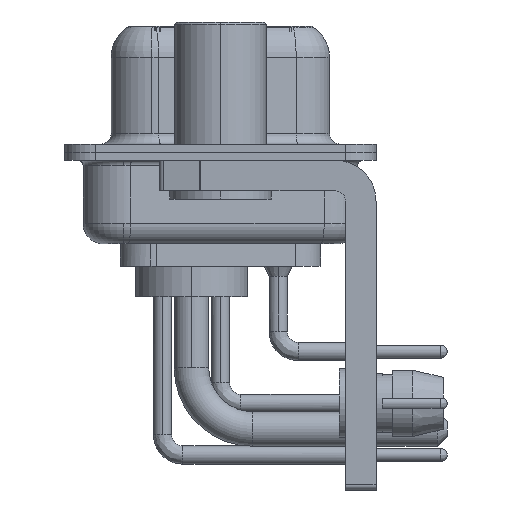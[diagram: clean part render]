
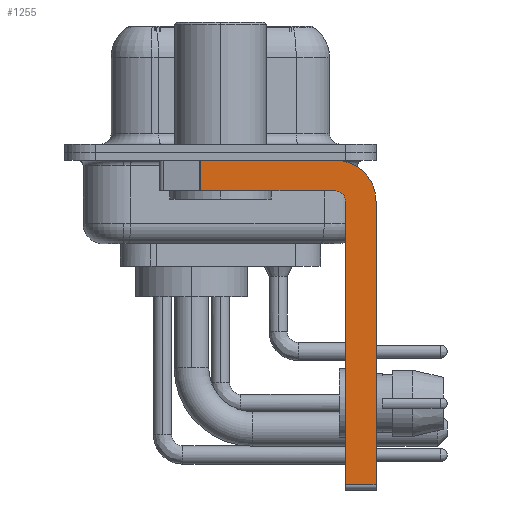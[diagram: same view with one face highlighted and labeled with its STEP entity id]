
A CAD part, left-side view. The second image highlights one B-rep face of the part: STEP entity #1255.
In plain terms, the highlighted planar face has unit normal (-1, 0, 0).
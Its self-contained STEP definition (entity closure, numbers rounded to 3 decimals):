
#630 = ORIENTED_EDGE ( 'NONE', *, *, #1553, .F. ) ;
#1255 = ADVANCED_FACE ( 'NONE', ( #2744 ), #27591, .F. ) ;
#1553 = EDGE_CURVE ( 'NONE', #31914, #4604, #4413, .T. ) ;
#1892 = CARTESIAN_POINT ( 'NONE',  ( -2.9, 0.978, -1.9 ) ) ;
#1980 = EDGE_CURVE ( 'NONE', #17099, #31914, #19887, .T. ) ;
#2428 = CARTESIAN_POINT ( 'NONE',  ( -2.9, 0.978, -0.4 ) ) ;
#2476 = LINE ( 'NONE', #30047, #4962 ) ;
#2685 = AXIS2_PLACEMENT_3D ( 'NONE', #12939, #18265, #9809 ) ;
#2696 = DIRECTION ( 'NONE',  ( 0., 0., -1. ) ) ;
#2702 = VECTOR ( 'NONE', #23407, 1000. ) ;
#2744 = FACE_OUTER_BOUND ( 'NONE', #30537, .T. ) ;
#4413 = CIRCLE ( 'NONE', #2685, 2. ) ;
#4604 = VERTEX_POINT ( 'NONE', #15969 ) ;
#4962 = VECTOR ( 'NONE', #35711, 1000. ) ;
#5064 = LINE ( 'NONE', #13667, #18791 ) ;
#5450 = ORIENTED_EDGE ( 'NONE', *, *, #23052, .F. ) ;
#5468 = EDGE_CURVE ( 'NONE', #18731, #22266, #2476, .T. ) ;
#5472 = DIRECTION ( 'NONE',  ( 0., 0., -1. ) ) ;
#5540 = EDGE_CURVE ( 'NONE', #31088, #14225, #25123, .T. ) ;
#5852 = ORIENTED_EDGE ( 'NONE', *, *, #6042, .F. ) ;
#5921 = DIRECTION ( 'NONE',  ( 0., -1., 0. ) ) ;
#5974 = CARTESIAN_POINT ( 'NONE',  ( -2.9, 3., -0.4 ) ) ;
#6042 = EDGE_CURVE ( 'NONE', #31088, #7208, #34734, .T. ) ;
#6273 = EDGE_CURVE ( 'NONE', #17099, #22266, #23935, .T. ) ;
#7134 = CARTESIAN_POINT ( 'NONE',  ( -2.9, -5.65, -1.9 ) ) ;
#7208 = VERTEX_POINT ( 'NONE', #22126 ) ;
#9035 = CARTESIAN_POINT ( 'NONE',  ( -2.9, -5.65, -16.35 ) ) ;
#9809 = DIRECTION ( 'NONE',  ( 0., 0., -1. ) ) ;
#10960 = CARTESIAN_POINT ( 'NONE',  ( -2.9, -6.15, -16.35 ) ) ;
#11982 = EDGE_CURVE ( 'NONE', #4604, #14225, #5064, .T. ) ;
#12939 = CARTESIAN_POINT ( 'NONE',  ( -2.9, -5.65, -2.4 ) ) ;
#13667 = CARTESIAN_POINT ( 'NONE',  ( -2.9, -7.65, -2.4 ) ) ;
#13763 = CARTESIAN_POINT ( 'NONE',  ( -2.9, -7.65, -16.35 ) ) ;
#14225 = VERTEX_POINT ( 'NONE', #13763 ) ;
#14446 = DIRECTION ( 'NONE',  ( 0., 0., 1. ) ) ;
#14724 = ORIENTED_EDGE ( 'NONE', *, *, #11982, .F. ) ;
#15969 = CARTESIAN_POINT ( 'NONE',  ( -2.9, -7.65, -2.4 ) ) ;
#17045 = ORIENTED_EDGE ( 'NONE', *, *, #5468, .F. ) ;
#17099 = VERTEX_POINT ( 'NONE', #2428 ) ;
#17955 = CARTESIAN_POINT ( 'NONE',  ( -2.9, -6.15, -16.6 ) ) ;
#18107 = ORIENTED_EDGE ( 'NONE', *, *, #1980, .F. ) ;
#18265 = DIRECTION ( 'NONE',  ( 1., 0., 0. ) ) ;
#18731 = VERTEX_POINT ( 'NONE', #7134 ) ;
#18791 = VECTOR ( 'NONE', #2696, 1000. ) ;
#19751 = DIRECTION ( 'NONE',  ( 1., 0., 0. ) ) ;
#19887 = LINE ( 'NONE', #5974, #26846 ) ;
#20798 = VECTOR ( 'NONE', #24302, 1000. ) ;
#21225 = CARTESIAN_POINT ( 'NONE',  ( -2.9, 0.978, -1.9 ) ) ;
#21958 = ORIENTED_EDGE ( 'NONE', *, *, #5540, .T. ) ;
#22126 = CARTESIAN_POINT ( 'NONE',  ( -2.9, -6.15, -2.4 ) ) ;
#22266 = VERTEX_POINT ( 'NONE', #1892 ) ;
#22480 = CARTESIAN_POINT ( 'NONE',  ( -2.9, -5.65, -2.4 ) ) ;
#23052 = EDGE_CURVE ( 'NONE', #7208, #18731, #32896, .T. ) ;
#23407 = DIRECTION ( 'NONE',  ( 0., 0., 1. ) ) ;
#23935 = LINE ( 'NONE', #21225, #20798 ) ;
#24302 = DIRECTION ( 'NONE',  ( 0., 0., -1. ) ) ;
#25123 = LINE ( 'NONE', #9035, #31268 ) ;
#26846 = VECTOR ( 'NONE', #31016, 1000. ) ;
#27591 = PLANE ( 'NONE',  #32417 ) ;
#28163 = ORIENTED_EDGE ( 'NONE', *, *, #6273, .T. ) ;
#28676 = DIRECTION ( 'NONE',  ( -1., 0., 0. ) ) ;
#29366 = AXIS2_PLACEMENT_3D ( 'NONE', #34178, #28676, #14446 ) ;
#30047 = CARTESIAN_POINT ( 'NONE',  ( -2.9, -5.65, -1.9 ) ) ;
#30537 = EDGE_LOOP ( 'NONE', ( #18107, #28163, #17045, #5450, #5852, #21958, #14724, #630 ) ) ;
#31016 = DIRECTION ( 'NONE',  ( 0., -1., 0. ) ) ;
#31088 = VERTEX_POINT ( 'NONE', #10960 ) ;
#31268 = VECTOR ( 'NONE', #5921, 1000. ) ;
#31914 = VERTEX_POINT ( 'NONE', #35156 ) ;
#32417 = AXIS2_PLACEMENT_3D ( 'NONE', #22480, #19751, #5472 ) ;
#32896 = CIRCLE ( 'NONE', #29366, 0.5 ) ;
#34178 = CARTESIAN_POINT ( 'NONE',  ( -2.9, -5.65, -2.4 ) ) ;
#34734 = LINE ( 'NONE', #17955, #2702 ) ;
#35156 = CARTESIAN_POINT ( 'NONE',  ( -2.9, -5.65, -0.4 ) ) ;
#35711 = DIRECTION ( 'NONE',  ( 0., 1., 0. ) ) ;
